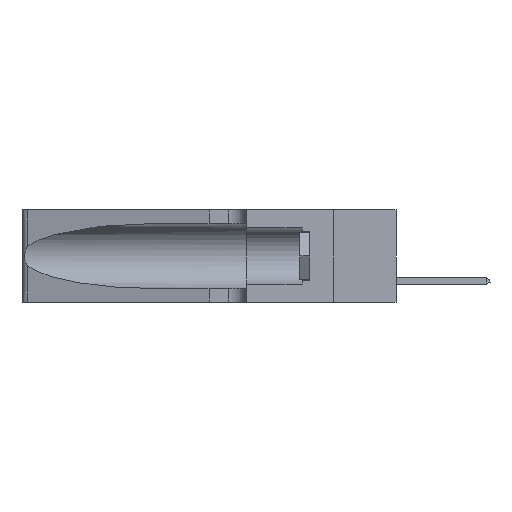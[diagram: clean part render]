
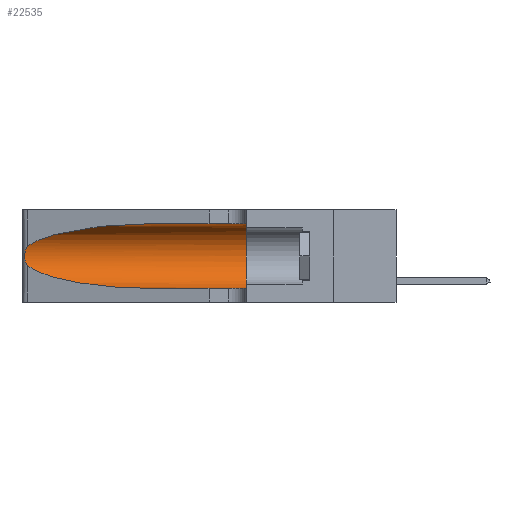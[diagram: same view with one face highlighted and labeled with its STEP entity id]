
A CAD part, left-side view. The second image highlights one B-rep face of the part: STEP entity #22535.
In plain terms, the highlighted cylindrical face has radius 3.308 mm (diameter 6.617 mm), a partial arc.
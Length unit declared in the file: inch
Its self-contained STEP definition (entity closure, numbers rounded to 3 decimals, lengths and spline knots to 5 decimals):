
#839 = ORIENTED_EDGE ( 'NONE', *, *, #33302, .T. ) ;
#2259 = CYLINDRICAL_SURFACE ( 'NONE', #32988, 0.13025 ) ;
#2342 = ORIENTED_EDGE ( 'NONE', *, *, #31203, .F. ) ;
#2392 = CARTESIAN_POINT ( 'NONE',  ( 0.2373, 1.15595, 0.28018 ) ) ;
#3588 = CARTESIAN_POINT ( 'NONE',  ( 0.26075, 1.23896, 0.19203 ) ) ;
#3713 = CARTESIAN_POINT ( 'NONE',  ( 0.26075, 1.23896, 0.178 ) ) ;
#4296 = CARTESIAN_POINT ( 'NONE',  ( 0.25639, 1.23186, 0.15144 ) ) ;
#5075 = CARTESIAN_POINT ( 'NONE',  ( 0.1305, 0.72297, 0.31525 ) ) ;
#5711 = DIRECTION ( 'NONE',  ( 0., -1., 0. ) ) ;
#6232 = CARTESIAN_POINT ( 'NONE',  ( 0.26018, 1.23835, 0.19895 ) ) ;
#6934 = CARTESIAN_POINT ( 'NONE',  ( 0.25555, 1.22994, 0.2215 ) ) ;
#7125 = ORIENTED_EDGE ( 'NONE', *, *, #16926, .F. ) ;
#7192 = CARTESIAN_POINT ( 'NONE',  ( 0.25789, 1.23486, 0.15765 ) ) ;
#7527 = VECTOR ( 'NONE', #27572, 39.37008 ) ;
#7760 = CARTESIAN_POINT ( 'NONE',  ( 0.25487, 1.22718, 0.14631 ) ) ;
#7769 = CARTESIAN_POINT ( 'NONE',  ( 0.25487, 1.22718, 0.14631 ) ) ;
#9303 = CARTESIAN_POINT ( 'NONE',  ( 0.25487, 1.22718, 0.14631 ) ) ;
#9715 = CARTESIAN_POINT ( 'NONE',  ( 0.1305, 0.35, 0.185 ) ) ;
#11176 = EDGE_CURVE ( 'NONE', #17708, #41050, #39534, .T. ) ;
#12330 =( BOUNDED_CURVE ( )  B_SPLINE_CURVE ( 3, ( #18704, #31770, #2392, #42214 ),
 .UNSPECIFIED., .F., .F. ) 
 B_SPLINE_CURVE_WITH_KNOTS ( ( 4, 4 ),
 ( 1.5708, 2.84003 ),
 .UNSPECIFIED. ) 
 CURVE ( )  GEOMETRIC_REPRESENTATION_ITEM ( )  RATIONAL_B_SPLINE_CURVE ( ( 1., 0.87, 0.87, 1. ) ) 
 REPRESENTATION_ITEM ( '' )  );
#14423 = CARTESIAN_POINT ( 'NONE',  ( 0.25555, 1.22993, 0.14849 ) ) ;
#15421 = CARTESIAN_POINT ( 'NONE',  ( 0.1305, 1.61858, 0.185 ) ) ;
#15955 = CARTESIAN_POINT ( 'NONE',  ( 0.18966, 0.96281, 0.05475 ) ) ;
#16926 = EDGE_CURVE ( 'NONE', #38993, #28457, #38127, .T. ) ;
#17385 = CARTESIAN_POINT ( 'NONE',  ( 0.25787, 1.23484, 0.2124 ) ) ;
#17708 = VERTEX_POINT ( 'NONE', #7769 ) ;
#18419 = EDGE_LOOP ( 'NONE', ( #26429, #839, #22547, #22122, #7125, #2342 ) ) ;
#18704 = CARTESIAN_POINT ( 'NONE',  ( 0.1305, 0.72297, 0.31525 ) ) ;
#20463 = LINE ( 'NONE', #29801, #22037 ) ;
#21538 = CARTESIAN_POINT ( 'NONE',  ( 0.1305, 0.72297, 0.05475 ) ) ;
#21555 = CARTESIAN_POINT ( 'NONE',  ( 0.1305, 0.35, 0.05475 ) ) ;
#22037 = VECTOR ( 'NONE', #30198, 39.37008 ) ;
#22122 = ORIENTED_EDGE ( 'NONE', *, *, #30055, .T. ) ;
#22535 = ADVANCED_FACE ( 'NONE', ( #42314 ), #2259, .F. ) ;
#22547 = ORIENTED_EDGE ( 'NONE', *, *, #11176, .T. ) ;
#22746 = LINE ( 'NONE', #27141, #7527 ) ;
#24756 = AXIS2_PLACEMENT_3D ( 'NONE', #9715, #42412, #32847 ) ;
#26010 = CARTESIAN_POINT ( 'NONE',  ( 0.1305, 0.35, 0.31525 ) ) ;
#26429 = ORIENTED_EDGE ( 'NONE', *, *, #30684, .T. ) ;
#27141 = CARTESIAN_POINT ( 'NONE',  ( 0.1305, 1.61858, 0.31525 ) ) ;
#27572 = DIRECTION ( 'NONE',  ( 0., -1., 0. ) ) ;
#27787 = B_SPLINE_CURVE_WITH_KNOTS ( 'NONE', 3,
 ( #35738, #6934, #29513, #17385, #40064, #6232, #3588, #3713, #36971, #40335, #7192, #4296, #14423, #7760 ),
 .UNSPECIFIED., .F., .F.,
 ( 4, 2, 2, 2, 2, 2, 4 ),
 ( 0., 0.00027, 0.00053, 0.00107, 0.0016, 0.00187, 0.00214 ),
 .UNSPECIFIED. ) ;
#28457 = VERTEX_POINT ( 'NONE', #21555 ) ;
#29513 = CARTESIAN_POINT ( 'NONE',  ( 0.25639, 1.23184, 0.21858 ) ) ;
#29801 = CARTESIAN_POINT ( 'NONE',  ( 0.1305, 1.61858, 0.05475 ) ) ;
#30055 = EDGE_CURVE ( 'NONE', #41050, #28457, #20463, .T. ) ;
#30198 = DIRECTION ( 'NONE',  ( 0., -1., 0. ) ) ;
#30684 = EDGE_CURVE ( 'NONE', #37390, #40768, #12330, .T. ) ;
#31203 = EDGE_CURVE ( 'NONE', #37390, #38993, #22746, .T. ) ;
#31578 = DIRECTION ( 'NONE',  ( 0., 0., -1. ) ) ;
#31770 = CARTESIAN_POINT ( 'NONE',  ( 0.18966, 0.96281, 0.31525 ) ) ;
#32586 = CARTESIAN_POINT ( 'NONE',  ( 0.2373, 1.15595, 0.08982 ) ) ;
#32847 = DIRECTION ( 'NONE',  ( 0., 0., 1. ) ) ;
#32988 = AXIS2_PLACEMENT_3D ( 'NONE', #15421, #5711, #31578 ) ;
#33302 = EDGE_CURVE ( 'NONE', #40768, #17708, #27787, .T. ) ;
#35738 = CARTESIAN_POINT ( 'NONE',  ( 0.25487, 1.22718, 0.22369 ) ) ;
#36971 = CARTESIAN_POINT ( 'NONE',  ( 0.26017, 1.23833, 0.17102 ) ) ;
#37390 = VERTEX_POINT ( 'NONE', #5075 ) ;
#38127 = CIRCLE ( 'NONE', #24756, 0.13025 ) ;
#38993 = VERTEX_POINT ( 'NONE', #26010 ) ;
#39534 =( BOUNDED_CURVE ( )  B_SPLINE_CURVE ( 3, ( #9303, #32586, #15955, #41173 ),
 .UNSPECIFIED., .F., .F. ) 
 B_SPLINE_CURVE_WITH_KNOTS ( ( 4, 4 ),
 ( 3.44316, 4.71239 ),
 .UNSPECIFIED. ) 
 CURVE ( )  GEOMETRIC_REPRESENTATION_ITEM ( )  RATIONAL_B_SPLINE_CURVE ( ( 1., 0.87, 0.87, 1. ) ) 
 REPRESENTATION_ITEM ( '' )  );
#40064 = CARTESIAN_POINT ( 'NONE',  ( 0.25854, 1.2359, 0.20912 ) ) ;
#40335 = CARTESIAN_POINT ( 'NONE',  ( 0.25856, 1.23593, 0.16098 ) ) ;
#40768 = VERTEX_POINT ( 'NONE', #42567 ) ;
#41050 = VERTEX_POINT ( 'NONE', #21538 ) ;
#41173 = CARTESIAN_POINT ( 'NONE',  ( 0.1305, 0.72297, 0.05475 ) ) ;
#42214 = CARTESIAN_POINT ( 'NONE',  ( 0.25487, 1.22718, 0.22369 ) ) ;
#42314 = FACE_OUTER_BOUND ( 'NONE', #18419, .T. ) ;
#42412 = DIRECTION ( 'NONE',  ( 0., 1., 0. ) ) ;
#42567 = CARTESIAN_POINT ( 'NONE',  ( 0.25487, 1.22718, 0.22369 ) ) ;
